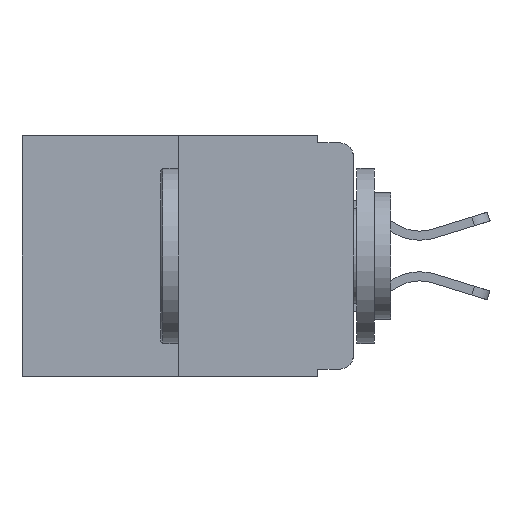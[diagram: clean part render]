
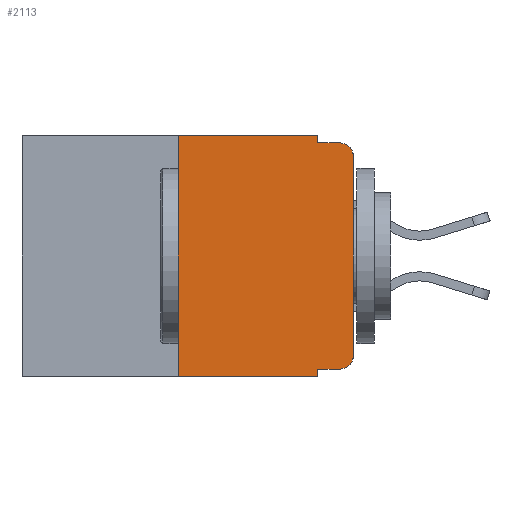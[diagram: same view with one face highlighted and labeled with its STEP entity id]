
A CAD part, left-side view. The second image highlights one B-rep face of the part: STEP entity #2113.
In plain terms, the highlighted planar face has unit normal (-1, 0, 0).
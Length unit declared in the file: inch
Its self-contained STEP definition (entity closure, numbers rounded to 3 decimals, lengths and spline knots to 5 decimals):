
#207 = VERTEX_POINT ( 'NONE', #11646 ) ;
#367 = VERTEX_POINT ( 'NONE', #10655 ) ;
#1000 = VERTEX_POINT ( 'NONE', #8164 ) ;
#1293 = AXIS2_PLACEMENT_3D ( 'NONE', #7001, #2059, #2018 ) ;
#1478 = LINE ( 'NONE', #2892, #8942 ) ;
#1621 = DIRECTION ( 'NONE',  ( 0., -1., 0. ) ) ;
#2018 = DIRECTION ( 'NONE',  ( 0., 0., -1. ) ) ;
#2042 = LINE ( 'NONE', #4549, #11994 ) ;
#2055 = LINE ( 'NONE', #4840, #3761 ) ;
#2059 = DIRECTION ( 'NONE',  ( 1., 0., 0. ) ) ;
#2113 = ADVANCED_FACE ( 'NONE', ( #4410 ), #9717, .F. ) ;
#2170 = CARTESIAN_POINT ( 'NONE',  ( 0., 0.473, 0. ) ) ;
#2240 = AXIS2_PLACEMENT_3D ( 'NONE', #7429, #7393, #2594 ) ;
#2594 = DIRECTION ( 'NONE',  ( 0., 0., -1. ) ) ;
#2595 = EDGE_CURVE ( 'NONE', #8769, #367, #6605, .T. ) ;
#2665 = CIRCLE ( 'NONE', #2240, 0.02 ) ;
#2892 = CARTESIAN_POINT ( 'NONE',  ( 0., 0.051, 0. ) ) ;
#2894 = AXIS2_PLACEMENT_3D ( 'NONE', #8949, #3367, #9910 ) ;
#2910 = EDGE_CURVE ( 'NONE', #1000, #11910, #9804, .T. ) ;
#3034 = ORIENTED_EDGE ( 'NONE', *, *, #7940, .T. ) ;
#3367 = DIRECTION ( 'NONE',  ( -1., 0., 0. ) ) ;
#3427 = VECTOR ( 'NONE', #12530, 39.37008 ) ;
#3506 = ORIENTED_EDGE ( 'NONE', *, *, #9059, .F. ) ;
#3761 = VECTOR ( 'NONE', #12407, 39.37008 ) ;
#3790 = ORIENTED_EDGE ( 'NONE', *, *, #5612, .T. ) ;
#3835 = LINE ( 'NONE', #8662, #6158 ) ;
#3896 = DIRECTION ( 'NONE',  ( 0., 0., -1. ) ) ;
#3926 = EDGE_CURVE ( 'NONE', #207, #4540, #2665, .T. ) ;
#4092 = DIRECTION ( 'NONE',  ( 0., -1., 0. ) ) ;
#4261 = VECTOR ( 'NONE', #1621, 39.37008 ) ;
#4343 = CARTESIAN_POINT ( 'NONE',  ( 0., 0.051, -0.333 ) ) ;
#4410 = FACE_OUTER_BOUND ( 'NONE', #7353, .T. ) ;
#4469 = VERTEX_POINT ( 'NONE', #12794 ) ;
#4540 = VERTEX_POINT ( 'NONE', #12567 ) ;
#4549 = CARTESIAN_POINT ( 'NONE',  ( 0., 0.051, 0. ) ) ;
#4650 = EDGE_CURVE ( 'NONE', #4469, #12201, #9339, .T. ) ;
#4840 = CARTESIAN_POINT ( 'NONE',  ( 0., 0., 0. ) ) ;
#4860 = ORIENTED_EDGE ( 'NONE', *, *, #10366, .F. ) ;
#4921 = CARTESIAN_POINT ( 'NONE',  ( 0., 0.051, -0.01 ) ) ;
#5006 = ORIENTED_EDGE ( 'NONE', *, *, #2595, .F. ) ;
#5612 = EDGE_CURVE ( 'NONE', #8540, #207, #2055, .T. ) ;
#6096 = EDGE_CURVE ( 'NONE', #367, #10112, #2042, .T. ) ;
#6158 = VECTOR ( 'NONE', #6672, 39.37008 ) ;
#6498 = CIRCLE ( 'NONE', #2894, 0.02 ) ;
#6605 = LINE ( 'NONE', #2170, #4261 ) ;
#6632 = CARTESIAN_POINT ( 'NONE',  ( 0., 0.051, -0.343 ) ) ;
#6672 = DIRECTION ( 'NONE',  ( 0., 0., 1. ) ) ;
#6698 = ORIENTED_EDGE ( 'NONE', *, *, #7782, .F. ) ;
#7001 = CARTESIAN_POINT ( 'NONE',  ( 0., 0.473, 0. ) ) ;
#7218 = VECTOR ( 'NONE', #4092, 39.37008 ) ;
#7353 = EDGE_LOOP ( 'NONE', ( #3790, #7756, #6698, #8710, #5006, #4860, #8237, #3506, #11763, #3034 ) ) ;
#7389 = CARTESIAN_POINT ( 'NONE',  ( 0., 0.473, -0.343 ) ) ;
#7393 = DIRECTION ( 'NONE',  ( -1., 0., 0. ) ) ;
#7429 = CARTESIAN_POINT ( 'NONE',  ( 0., 0.02, -0.03 ) ) ;
#7756 = ORIENTED_EDGE ( 'NONE', *, *, #3926, .T. ) ;
#7782 = EDGE_CURVE ( 'NONE', #10112, #4540, #8327, .T. ) ;
#7940 = EDGE_CURVE ( 'NONE', #12201, #8540, #6498, .T. ) ;
#8164 = CARTESIAN_POINT ( 'NONE',  ( 0., 0.25, -0.343 ) ) ;
#8237 = ORIENTED_EDGE ( 'NONE', *, *, #2910, .T. ) ;
#8327 = LINE ( 'NONE', #4921, #3427 ) ;
#8540 = VERTEX_POINT ( 'NONE', #8802 ) ;
#8662 = CARTESIAN_POINT ( 'NONE',  ( 0., 0.25, 0. ) ) ;
#8710 = ORIENTED_EDGE ( 'NONE', *, *, #6096, .F. ) ;
#8769 = VERTEX_POINT ( 'NONE', #9107 ) ;
#8802 = CARTESIAN_POINT ( 'NONE',  ( 0., 0., -0.313 ) ) ;
#8942 = VECTOR ( 'NONE', #3896, 39.37008 ) ;
#8949 = CARTESIAN_POINT ( 'NONE',  ( 0., 0.02, -0.313 ) ) ;
#9044 = VECTOR ( 'NONE', #9964, 39.37008 ) ;
#9059 = EDGE_CURVE ( 'NONE', #4469, #11910, #1478, .T. ) ;
#9107 = CARTESIAN_POINT ( 'NONE',  ( 0., 0.25, 0. ) ) ;
#9257 = DIRECTION ( 'NONE',  ( 0., 0., -1. ) ) ;
#9339 = LINE ( 'NONE', #4343, #9044 ) ;
#9717 = PLANE ( 'NONE',  #1293 ) ;
#9804 = LINE ( 'NONE', #7389, #7218 ) ;
#9910 = DIRECTION ( 'NONE',  ( 0., 0., -1. ) ) ;
#9964 = DIRECTION ( 'NONE',  ( 0., -1., 0. ) ) ;
#10112 = VERTEX_POINT ( 'NONE', #12166 ) ;
#10366 = EDGE_CURVE ( 'NONE', #1000, #8769, #3835, .T. ) ;
#10655 = CARTESIAN_POINT ( 'NONE',  ( 0., 0.051, 0. ) ) ;
#11646 = CARTESIAN_POINT ( 'NONE',  ( 0., 0., -0.03 ) ) ;
#11763 = ORIENTED_EDGE ( 'NONE', *, *, #4650, .T. ) ;
#11910 = VERTEX_POINT ( 'NONE', #6632 ) ;
#11949 = CARTESIAN_POINT ( 'NONE',  ( 0., 0.02, -0.333 ) ) ;
#11994 = VECTOR ( 'NONE', #9257, 39.37008 ) ;
#12166 = CARTESIAN_POINT ( 'NONE',  ( 0., 0.051, -0.01 ) ) ;
#12201 = VERTEX_POINT ( 'NONE', #11949 ) ;
#12407 = DIRECTION ( 'NONE',  ( 0., 0., 1. ) ) ;
#12530 = DIRECTION ( 'NONE',  ( 0., -1., 0. ) ) ;
#12567 = CARTESIAN_POINT ( 'NONE',  ( 0., 0.02, -0.01 ) ) ;
#12794 = CARTESIAN_POINT ( 'NONE',  ( 0., 0.051, -0.333 ) ) ;
